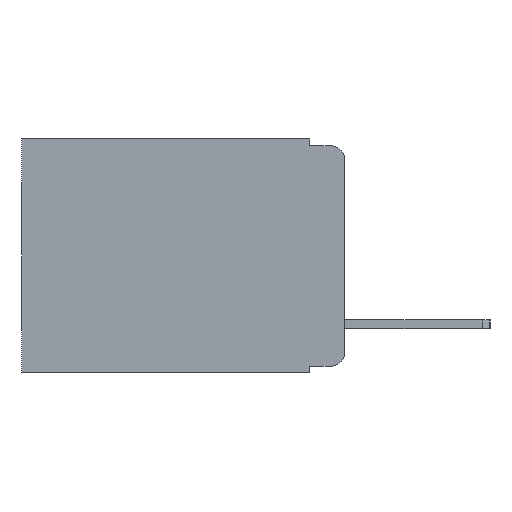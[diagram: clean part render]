
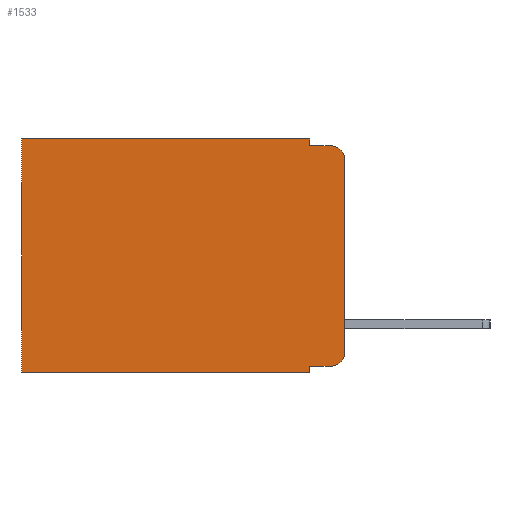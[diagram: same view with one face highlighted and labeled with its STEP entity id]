
A CAD part, left-side view. The second image highlights one B-rep face of the part: STEP entity #1533.
In plain terms, the highlighted planar face has unit normal (-1, 0, 0).
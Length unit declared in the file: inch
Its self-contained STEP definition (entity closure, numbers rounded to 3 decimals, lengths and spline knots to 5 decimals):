
#32 = DIRECTION ( 'NONE',  ( -1., 0., 0. ) ) ;
#343 = ORIENTED_EDGE ( 'NONE', *, *, #4139, .F. ) ;
#605 = VECTOR ( 'NONE', #2844, 39.37008 ) ;
#637 = DIRECTION ( 'NONE',  ( -1., 0., 0. ) ) ;
#713 = DIRECTION ( 'NONE',  ( 0., 0., -1. ) ) ;
#961 = ORIENTED_EDGE ( 'NONE', *, *, #2505, .F. ) ;
#968 = CARTESIAN_POINT ( 'NONE',  ( 0.298, 0.02, -0.01 ) ) ;
#1247 = AXIS2_PLACEMENT_3D ( 'NONE', #6019, #637, #6871 ) ;
#1337 = CARTESIAN_POINT ( 'NONE',  ( 0.298, 0.051, -0.343 ) ) ;
#1367 = PLANE ( 'NONE',  #2218 ) ;
#1533 = ADVANCED_FACE ( 'NONE', ( #3761 ), #1367, .F. ) ;
#1560 = EDGE_CURVE ( 'NONE', #5910, #8194, #6542, .T. ) ;
#1788 = VERTEX_POINT ( 'NONE', #5728 ) ;
#1946 = DIRECTION ( 'NONE',  ( 0., -1., 0. ) ) ;
#1997 = DIRECTION ( 'NONE',  ( 0., 0., -1. ) ) ;
#2099 = VERTEX_POINT ( 'NONE', #9709 ) ;
#2189 = VERTEX_POINT ( 'NONE', #1337 ) ;
#2218 = AXIS2_PLACEMENT_3D ( 'NONE', #4928, #2327, #8310 ) ;
#2327 = DIRECTION ( 'NONE',  ( 1., 0., 0. ) ) ;
#2505 = EDGE_CURVE ( 'NONE', #6987, #2189, #10046, .T. ) ;
#2519 = EDGE_CURVE ( 'NONE', #6987, #9741, #3490, .T. ) ;
#2523 = EDGE_CURVE ( 'NONE', #9741, #3930, #5453, .T. ) ;
#2753 = VECTOR ( 'NONE', #713, 39.37008 ) ;
#2844 = DIRECTION ( 'NONE',  ( 0., 1., 0. ) ) ;
#2920 = CARTESIAN_POINT ( 'NONE',  ( 0.298, 0.051, -0.333 ) ) ;
#3066 = LINE ( 'NONE', #3616, #2753 ) ;
#3161 = VECTOR ( 'NONE', #4752, 39.37008 ) ;
#3205 = VECTOR ( 'NONE', #1946, 39.37008 ) ;
#3216 = ORIENTED_EDGE ( 'NONE', *, *, #10599, .T. ) ;
#3467 = LINE ( 'NONE', #10308, #605 ) ;
#3490 = LINE ( 'NONE', #2920, #3205 ) ;
#3583 = VECTOR ( 'NONE', #8382, 39.37008 ) ;
#3616 = CARTESIAN_POINT ( 'NONE',  ( 0.298, 0.051, 0. ) ) ;
#3761 = FACE_OUTER_BOUND ( 'NONE', #6290, .T. ) ;
#3792 = ORIENTED_EDGE ( 'NONE', *, *, #2519, .T. ) ;
#3881 = CARTESIAN_POINT ( 'NONE',  ( 0.298, 0., -0.03 ) ) ;
#3930 = VERTEX_POINT ( 'NONE', #7953 ) ;
#3977 = VECTOR ( 'NONE', #8116, 39.37008 ) ;
#4025 = EDGE_CURVE ( 'NONE', #5910, #3930, #6741, .T. ) ;
#4139 = EDGE_CURVE ( 'NONE', #10515, #8194, #10008, .T. ) ;
#4413 = EDGE_CURVE ( 'NONE', #2189, #7814, #8302, .T. ) ;
#4752 = DIRECTION ( 'NONE',  ( 0., -1., 0. ) ) ;
#4928 = CARTESIAN_POINT ( 'NONE',  ( 0.298, 0., 0. ) ) ;
#4997 = CARTESIAN_POINT ( 'NONE',  ( 0.298, 0., -0.343 ) ) ;
#5453 = CIRCLE ( 'NONE', #7810, 0.02 ) ;
#5469 = ORIENTED_EDGE ( 'NONE', *, *, #6563, .T. ) ;
#5485 = CARTESIAN_POINT ( 'NONE',  ( 0.298, 0.02, -0.313 ) ) ;
#5490 = CARTESIAN_POINT ( 'NONE',  ( 0.298, 0., 0. ) ) ;
#5568 = CARTESIAN_POINT ( 'NONE',  ( 0.298, 0.473, 0. ) ) ;
#5728 = CARTESIAN_POINT ( 'NONE',  ( 0.298, 0.473, 0. ) ) ;
#5910 = VERTEX_POINT ( 'NONE', #3881 ) ;
#6019 = CARTESIAN_POINT ( 'NONE',  ( 0.298, 0.02, -0.03 ) ) ;
#6290 = EDGE_LOOP ( 'NONE', ( #9092, #9320, #343, #9566, #3216, #5469, #9797, #961, #3792, #8233 ) ) ;
#6339 = DIRECTION ( 'NONE',  ( 0., 0., -1. ) ) ;
#6542 = CIRCLE ( 'NONE', #1247, 0.02 ) ;
#6563 = EDGE_CURVE ( 'NONE', #1788, #7814, #10349, .T. ) ;
#6741 = LINE ( 'NONE', #5490, #10776 ) ;
#6871 = DIRECTION ( 'NONE',  ( 0., 0., -1. ) ) ;
#6987 = VERTEX_POINT ( 'NONE', #8857 ) ;
#7810 = AXIS2_PLACEMENT_3D ( 'NONE', #5485, #32, #6339 ) ;
#7814 = VERTEX_POINT ( 'NONE', #10093 ) ;
#7953 = CARTESIAN_POINT ( 'NONE',  ( 0.298, 0., -0.313 ) ) ;
#7985 = VECTOR ( 'NONE', #8761, 39.37008 ) ;
#8116 = DIRECTION ( 'NONE',  ( 0., 0., -1. ) ) ;
#8146 = CARTESIAN_POINT ( 'NONE',  ( 0.298, 0.051, -0.01 ) ) ;
#8194 = VERTEX_POINT ( 'NONE', #968 ) ;
#8233 = ORIENTED_EDGE ( 'NONE', *, *, #2523, .T. ) ;
#8302 = LINE ( 'NONE', #4997, #3583 ) ;
#8310 = DIRECTION ( 'NONE',  ( 0., 0., -1. ) ) ;
#8382 = DIRECTION ( 'NONE',  ( 0., 1., 0. ) ) ;
#8761 = DIRECTION ( 'NONE',  ( 0., 0., -1. ) ) ;
#8857 = CARTESIAN_POINT ( 'NONE',  ( 0.298, 0.051, -0.333 ) ) ;
#9092 = ORIENTED_EDGE ( 'NONE', *, *, #4025, .F. ) ;
#9320 = ORIENTED_EDGE ( 'NONE', *, *, #1560, .T. ) ;
#9566 = ORIENTED_EDGE ( 'NONE', *, *, #9986, .F. ) ;
#9709 = CARTESIAN_POINT ( 'NONE',  ( 0.298, 0.051, 0. ) ) ;
#9741 = VERTEX_POINT ( 'NONE', #9885 ) ;
#9797 = ORIENTED_EDGE ( 'NONE', *, *, #4413, .F. ) ;
#9885 = CARTESIAN_POINT ( 'NONE',  ( 0.298, 0.02, -0.333 ) ) ;
#9986 = EDGE_CURVE ( 'NONE', #2099, #10515, #3066, .T. ) ;
#10008 = LINE ( 'NONE', #8146, #3161 ) ;
#10046 = LINE ( 'NONE', #10301, #7985 ) ;
#10093 = CARTESIAN_POINT ( 'NONE',  ( 0.298, 0.473, -0.343 ) ) ;
#10301 = CARTESIAN_POINT ( 'NONE',  ( 0.298, 0.051, 0. ) ) ;
#10308 = CARTESIAN_POINT ( 'NONE',  ( 0.298, 0., 0. ) ) ;
#10349 = LINE ( 'NONE', #5568, #3977 ) ;
#10515 = VERTEX_POINT ( 'NONE', #10960 ) ;
#10599 = EDGE_CURVE ( 'NONE', #2099, #1788, #3467, .T. ) ;
#10776 = VECTOR ( 'NONE', #1997, 39.37008 ) ;
#10960 = CARTESIAN_POINT ( 'NONE',  ( 0.298, 0.051, -0.01 ) ) ;
